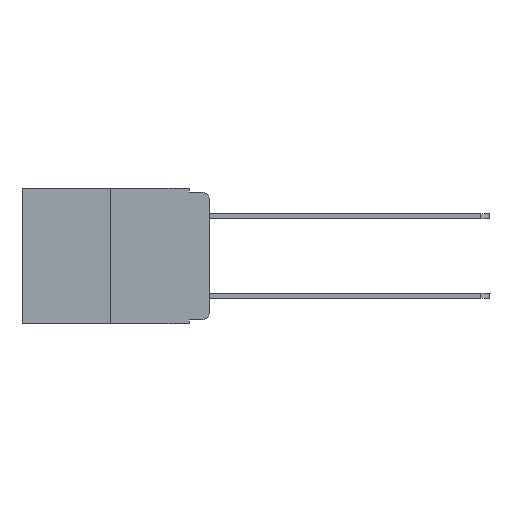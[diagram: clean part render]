
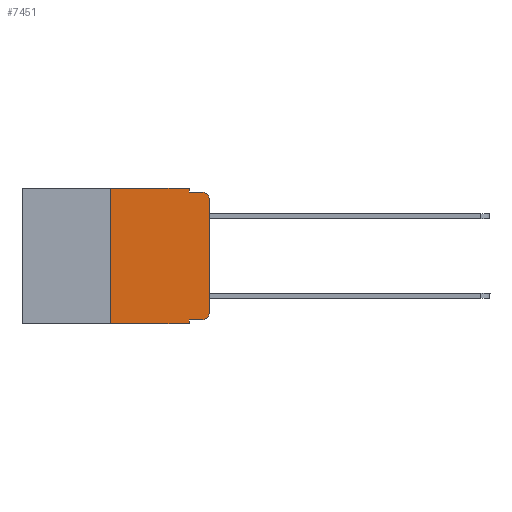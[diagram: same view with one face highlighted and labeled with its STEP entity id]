
A CAD part, left-side view. The second image highlights one B-rep face of the part: STEP entity #7451.
In plain terms, the highlighted planar face has unit normal (-1, 0, 0).
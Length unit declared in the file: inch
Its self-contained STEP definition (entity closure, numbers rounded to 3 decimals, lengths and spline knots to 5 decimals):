
#350 = VERTEX_POINT ( 'NONE', #6439 ) ;
#775 = LINE ( 'NONE', #12547, #1211 ) ;
#1211 = VECTOR ( 'NONE', #12923, 39.37008 ) ;
#1289 = CIRCLE ( 'NONE', #4632, 0.02 ) ;
#1524 = PLANE ( 'NONE',  #12566 ) ;
#1548 = LINE ( 'NONE', #20849, #17899 ) ;
#1650 = VECTOR ( 'NONE', #3139, 39.37008 ) ;
#2031 = VERTEX_POINT ( 'NONE', #6125 ) ;
#2117 = EDGE_LOOP ( 'NONE', ( #15691, #15207, #3514, #3846, #12925, #4029, #19819, #9690, #11686, #12963 ) ) ;
#2791 = CARTESIAN_POINT ( 'NONE',  ( 0., 0.02, -0.01 ) ) ;
#3139 = DIRECTION ( 'NONE',  ( 0., 0., 1. ) ) ;
#3514 = ORIENTED_EDGE ( 'NONE', *, *, #5799, .F. ) ;
#3846 = ORIENTED_EDGE ( 'NONE', *, *, #6550, .F. ) ;
#3942 = LINE ( 'NONE', #23889, #18463 ) ;
#4029 = ORIENTED_EDGE ( 'NONE', *, *, #17388, .F. ) ;
#4119 = VERTEX_POINT ( 'NONE', #11442 ) ;
#4581 = DIRECTION ( 'NONE',  ( -1., 0., 0. ) ) ;
#4632 = AXIS2_PLACEMENT_3D ( 'NONE', #7422, #25431, #15514 ) ;
#4638 = CARTESIAN_POINT ( 'NONE',  ( 0., 0.051, 0. ) ) ;
#5137 = LINE ( 'NONE', #21788, #24610 ) ;
#5667 = EDGE_CURVE ( 'NONE', #24476, #4119, #775, .T. ) ;
#5799 = EDGE_CURVE ( 'NONE', #17704, #10153, #1548, .T. ) ;
#5961 = CARTESIAN_POINT ( 'NONE',  ( 0., 0.051, 0. ) ) ;
#6125 = CARTESIAN_POINT ( 'NONE',  ( 0., 0., -0.03 ) ) ;
#6155 = DIRECTION ( 'NONE',  ( 0., -1., 0. ) ) ;
#6439 = CARTESIAN_POINT ( 'NONE',  ( 0., 0.25, 0. ) ) ;
#6550 = EDGE_CURVE ( 'NONE', #9924, #17704, #24461, .T. ) ;
#7159 = CARTESIAN_POINT ( 'NONE',  ( 0., 0.051, -0.333 ) ) ;
#7422 = CARTESIAN_POINT ( 'NONE',  ( 0., 0.02, -0.313 ) ) ;
#7451 = ADVANCED_FACE ( 'NONE', ( #23447 ), #1524, .F. ) ;
#7458 = EDGE_CURVE ( 'NONE', #21302, #23617, #1289, .T. ) ;
#7505 = AXIS2_PLACEMENT_3D ( 'NONE', #22437, #4581, #12558 ) ;
#9021 = CARTESIAN_POINT ( 'NONE',  ( 0., 0.051, -0.01 ) ) ;
#9156 = CARTESIAN_POINT ( 'NONE',  ( 0., 0., 0. ) ) ;
#9557 = VERTEX_POINT ( 'NONE', #11149 ) ;
#9690 = ORIENTED_EDGE ( 'NONE', *, *, #16494, .F. ) ;
#9924 = VERTEX_POINT ( 'NONE', #5961 ) ;
#10153 = VERTEX_POINT ( 'NONE', #2791 ) ;
#11149 = CARTESIAN_POINT ( 'NONE',  ( 0., 0.051, -0.333 ) ) ;
#11159 = EDGE_CURVE ( 'NONE', #9557, #21302, #15236, .T. ) ;
#11442 = CARTESIAN_POINT ( 'NONE',  ( 0., 0.051, -0.343 ) ) ;
#11608 = DIRECTION ( 'NONE',  ( 0., 0., -1. ) ) ;
#11673 = VECTOR ( 'NONE', #11608, 39.37008 ) ;
#11686 = ORIENTED_EDGE ( 'NONE', *, *, #11159, .T. ) ;
#12547 = CARTESIAN_POINT ( 'NONE',  ( 0., 0.473, -0.343 ) ) ;
#12558 = DIRECTION ( 'NONE',  ( 0., 0., -1. ) ) ;
#12566 = AXIS2_PLACEMENT_3D ( 'NONE', #20960, #17204, #15372 ) ;
#12616 = DIRECTION ( 'NONE',  ( 0., 0., -1. ) ) ;
#12628 = CARTESIAN_POINT ( 'NONE',  ( 0., 0.25, -0.343 ) ) ;
#12923 = DIRECTION ( 'NONE',  ( 0., -1., 0. ) ) ;
#12925 = ORIENTED_EDGE ( 'NONE', *, *, #21355, .F. ) ;
#12963 = ORIENTED_EDGE ( 'NONE', *, *, #7458, .T. ) ;
#14182 = VECTOR ( 'NONE', #12616, 39.37008 ) ;
#14247 = CARTESIAN_POINT ( 'NONE',  ( 0., 0.02, -0.333 ) ) ;
#14447 = EDGE_CURVE ( 'NONE', #2031, #10153, #19979, .T. ) ;
#14527 = EDGE_CURVE ( 'NONE', #23617, #2031, #16979, .T. ) ;
#15207 = ORIENTED_EDGE ( 'NONE', *, *, #14447, .T. ) ;
#15236 = LINE ( 'NONE', #7159, #20200 ) ;
#15372 = DIRECTION ( 'NONE',  ( 0., 0., -1. ) ) ;
#15514 = DIRECTION ( 'NONE',  ( 0., 0., -1. ) ) ;
#15691 = ORIENTED_EDGE ( 'NONE', *, *, #14527, .T. ) ;
#16494 = EDGE_CURVE ( 'NONE', #9557, #4119, #25310, .T. ) ;
#16979 = LINE ( 'NONE', #9156, #1650 ) ;
#17204 = DIRECTION ( 'NONE',  ( 1., 0., 0. ) ) ;
#17388 = EDGE_CURVE ( 'NONE', #24476, #350, #5137, .T. ) ;
#17704 = VERTEX_POINT ( 'NONE', #9021 ) ;
#17899 = VECTOR ( 'NONE', #25192, 39.37008 ) ;
#18463 = VECTOR ( 'NONE', #6155, 39.37008 ) ;
#19819 = ORIENTED_EDGE ( 'NONE', *, *, #5667, .T. ) ;
#19979 = CIRCLE ( 'NONE', #7505, 0.02 ) ;
#20013 = CARTESIAN_POINT ( 'NONE',  ( 0., 0., -0.313 ) ) ;
#20200 = VECTOR ( 'NONE', #23183, 39.37008 ) ;
#20849 = CARTESIAN_POINT ( 'NONE',  ( 0., 0.051, -0.01 ) ) ;
#20960 = CARTESIAN_POINT ( 'NONE',  ( 0., 0.473, 0. ) ) ;
#21287 = DIRECTION ( 'NONE',  ( 0., 0., 1. ) ) ;
#21302 = VERTEX_POINT ( 'NONE', #14247 ) ;
#21355 = EDGE_CURVE ( 'NONE', #350, #9924, #3942, .T. ) ;
#21788 = CARTESIAN_POINT ( 'NONE',  ( 0., 0.25, 0. ) ) ;
#22437 = CARTESIAN_POINT ( 'NONE',  ( 0., 0.02, -0.03 ) ) ;
#23183 = DIRECTION ( 'NONE',  ( 0., -1., 0. ) ) ;
#23447 = FACE_OUTER_BOUND ( 'NONE', #2117, .T. ) ;
#23617 = VERTEX_POINT ( 'NONE', #20013 ) ;
#23889 = CARTESIAN_POINT ( 'NONE',  ( 0., 0.473, 0. ) ) ;
#24461 = LINE ( 'NONE', #4638, #14182 ) ;
#24476 = VERTEX_POINT ( 'NONE', #12628 ) ;
#24610 = VECTOR ( 'NONE', #21287, 39.37008 ) ;
#25192 = DIRECTION ( 'NONE',  ( 0., -1., 0. ) ) ;
#25310 = LINE ( 'NONE', #25720, #11673 ) ;
#25431 = DIRECTION ( 'NONE',  ( -1., 0., 0. ) ) ;
#25720 = CARTESIAN_POINT ( 'NONE',  ( 0., 0.051, 0. ) ) ;
